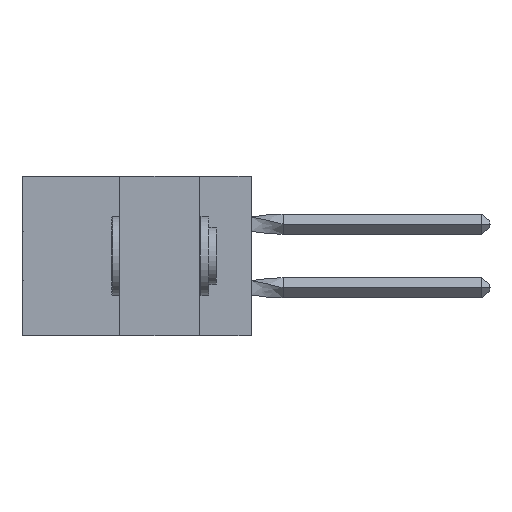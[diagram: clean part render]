
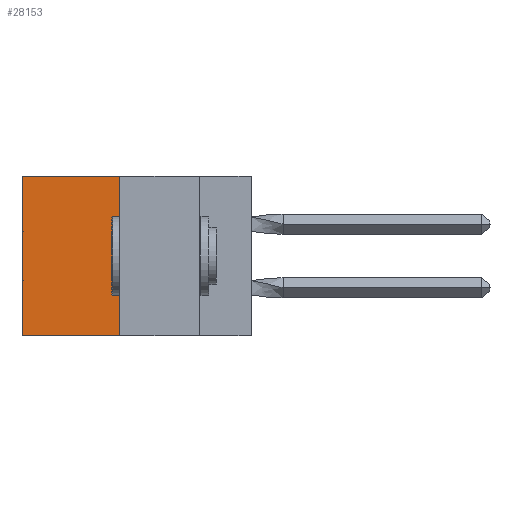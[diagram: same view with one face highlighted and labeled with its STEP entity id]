
A CAD part, left-side view. The second image highlights one B-rep face of the part: STEP entity #28153.
In plain terms, the highlighted planar face has unit normal (-1, 0, 0).
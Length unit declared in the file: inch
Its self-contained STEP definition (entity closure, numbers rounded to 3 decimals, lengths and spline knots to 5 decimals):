
#1169 = CARTESIAN_POINT ( 'NONE',  ( 0.305, 0.413, -0.5 ) ) ;
#2273 = LINE ( 'NONE', #7715, #19787 ) ;
#3933 = DIRECTION ( 'NONE',  ( 0., 1., 0. ) ) ;
#5130 = LINE ( 'NONE', #37745, #19767 ) ;
#5304 = CARTESIAN_POINT ( 'NONE',  ( 0.305, 0.413, -0.5 ) ) ;
#7715 = CARTESIAN_POINT ( 'NONE',  ( 0.305, 0.72, -0.5 ) ) ;
#8911 = DIRECTION ( 'NONE',  ( 0., 0., -1. ) ) ;
#9567 = CARTESIAN_POINT ( 'NONE',  ( 0.305, 0.72, 0. ) ) ;
#10930 = VERTEX_POINT ( 'NONE', #5304 ) ;
#12721 = ORIENTED_EDGE ( 'NONE', *, *, #16278, .T. ) ;
#14622 = EDGE_CURVE ( 'NONE', #39920, #10930, #44767, .T. ) ;
#16278 = EDGE_CURVE ( 'NONE', #39920, #43170, #20104, .T. ) ;
#19268 = CARTESIAN_POINT ( 'NONE',  ( 0.305, 0.413, -0.5 ) ) ;
#19767 = VECTOR ( 'NONE', #3933, 39.37008 ) ;
#19787 = VECTOR ( 'NONE', #33317, 39.37008 ) ;
#20104 = LINE ( 'NONE', #39230, #42266 ) ;
#21004 = ORIENTED_EDGE ( 'NONE', *, *, #14622, .F. ) ;
#23860 = EDGE_LOOP ( 'NONE', ( #44838, #34243, #21004, #12721 ) ) ;
#24748 = FACE_OUTER_BOUND ( 'NONE', #23860, .T. ) ;
#24994 = VECTOR ( 'NONE', #8911, 39.37008 ) ;
#26593 = DIRECTION ( 'NONE',  ( 1., 0., 0. ) ) ;
#28153 = ADVANCED_FACE ( 'NONE', ( #24748 ), #41458, .F. ) ;
#28233 = DIRECTION ( 'NONE',  ( 0., 1., 0. ) ) ;
#28561 = VERTEX_POINT ( 'NONE', #29355 ) ;
#29355 = CARTESIAN_POINT ( 'NONE',  ( 0.305, 0.72, -0.5 ) ) ;
#31651 = EDGE_CURVE ( 'NONE', #43170, #28561, #2273, .T. ) ;
#33317 = DIRECTION ( 'NONE',  ( 0., 0., -1. ) ) ;
#34243 = ORIENTED_EDGE ( 'NONE', *, *, #41522, .F. ) ;
#37745 = CARTESIAN_POINT ( 'NONE',  ( 0.305, 0.413, -0.5 ) ) ;
#39230 = CARTESIAN_POINT ( 'NONE',  ( 0.305, 0.413, 0. ) ) ;
#39785 = AXIS2_PLACEMENT_3D ( 'NONE', #19268, #26593, #44700 ) ;
#39920 = VERTEX_POINT ( 'NONE', #48041 ) ;
#41458 = PLANE ( 'NONE',  #39785 ) ;
#41522 = EDGE_CURVE ( 'NONE', #10930, #28561, #5130, .T. ) ;
#42266 = VECTOR ( 'NONE', #28233, 39.37008 ) ;
#43170 = VERTEX_POINT ( 'NONE', #9567 ) ;
#44700 = DIRECTION ( 'NONE',  ( 0., 0., -1. ) ) ;
#44767 = LINE ( 'NONE', #1169, #24994 ) ;
#44838 = ORIENTED_EDGE ( 'NONE', *, *, #31651, .T. ) ;
#48041 = CARTESIAN_POINT ( 'NONE',  ( 0.305, 0.413, 0. ) ) ;
